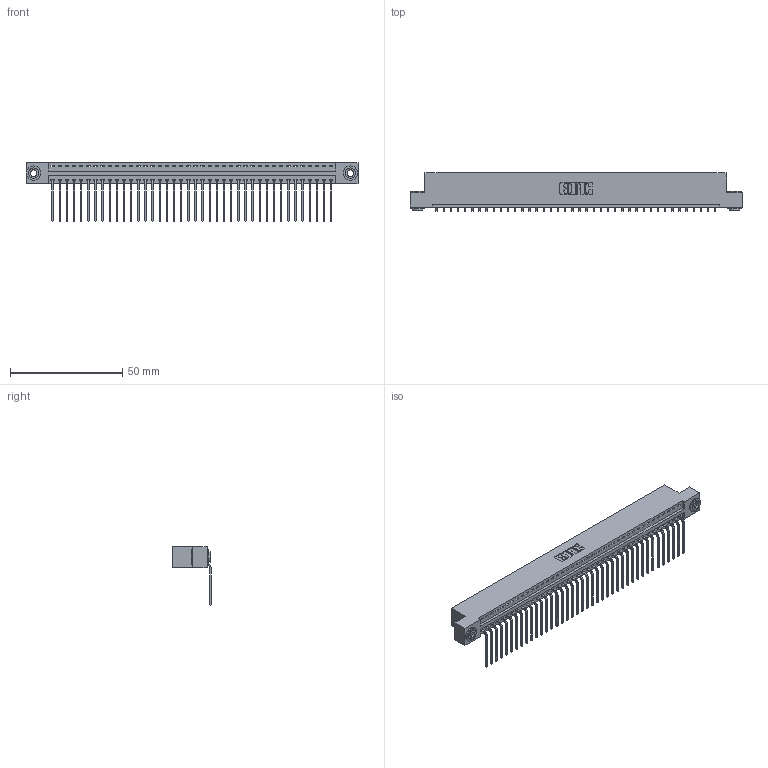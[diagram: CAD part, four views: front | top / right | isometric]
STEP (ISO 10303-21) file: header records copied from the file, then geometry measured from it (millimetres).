
FILE_DESCRIPTION (( 'STEP AP203' ), '1' );
FILE_NAME ('396-040-559-103.STEP', '2018-09-06T21:49:12', ( '' ), ( '' ), 'SwSTEP 2.0', 'SolidWorks 2016', '' );
FILE_SCHEMA (( 'CONFIG_CONTROL_DESIGN' ));
Length unit declared in the file: inch
Products named in the file (4): 346 Part_Flush Mounting Lugs - 0.156 Dia-TH; 396-040-559-103; 345-292-001_558 559 Tail - 1; 345-250-002_345-250-002-102
Assembly tree (43 placements, depth 2):
  396-040-559-103
    346 Part_Flush Mounting Lugs - 0.156 Dia-TH
    345-292-001_558 559 Tail - 1  x40
    345-250-002_345-250-002-102  x2
Bounding box: 147.57 x 17.08 x 26.16 mm (x, y, z)
Volume: 14265 mm3; surface area: 18822 mm2
Topology: 43 solids, 43 shells, 2560 faces, 7685 edges, 5066 vertices
Faces by surface type: plane 1766, cylinder 786, cone 8
Entity records: 25828 total; most frequent: CARTESIAN_POINT 4407, ORIENTED_EDGE 4374, DIRECTION 3921, EDGE_CURVE 2187, LINE 1871, VECTOR 1871, VERTEX_POINT 1454, AXIS2_PLACEMENT_3D 1025
